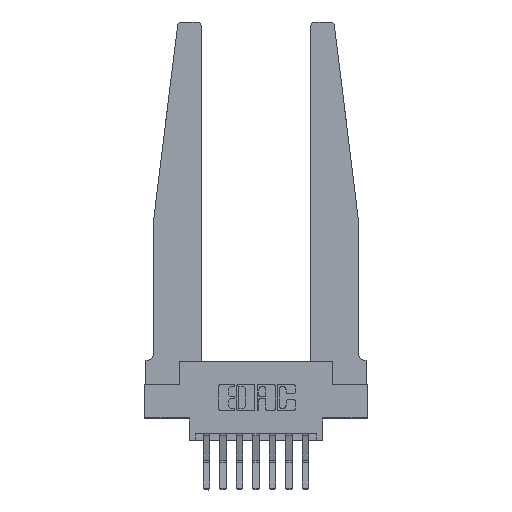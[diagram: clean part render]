
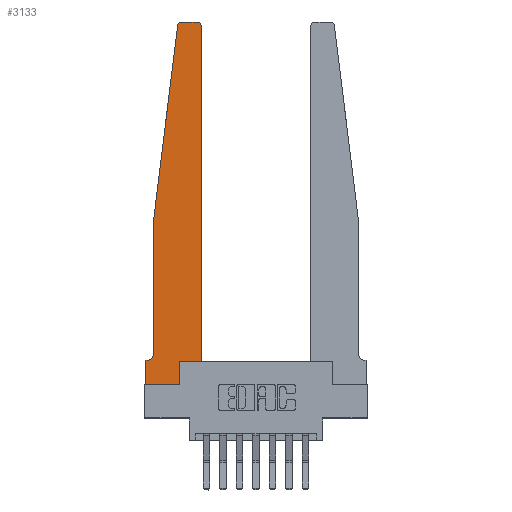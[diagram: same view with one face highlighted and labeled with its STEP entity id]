
A CAD part, top view. The second image highlights one B-rep face of the part: STEP entity #3133.
In plain terms, the highlighted planar face has unit normal (0, 0, 1).
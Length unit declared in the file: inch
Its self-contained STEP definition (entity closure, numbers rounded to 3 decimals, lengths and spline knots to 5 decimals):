
#712 = EDGE_CURVE ( 'NONE', #3959, #6302, #6384, .T. ) ;
#807 = CARTESIAN_POINT ( 'NONE',  ( 0.27653, 2.75, 0.37 ) ) ;
#1016 = CARTESIAN_POINT ( 'NONE',  ( 0.065, 0.2375, 0.37 ) ) ;
#1052 = DIRECTION ( 'NONE',  ( 1., 0., 0. ) ) ;
#1242 = LINE ( 'NONE', #12144, #10127 ) ;
#1416 = VERTEX_POINT ( 'NONE', #8526 ) ;
#1556 = VECTOR ( 'NONE', #14235, 39.37008 ) ;
#1967 = AXIS2_PLACEMENT_3D ( 'NONE', #14248, #7748, #1052 ) ;
#2050 = EDGE_CURVE ( 'NONE', #9724, #7909, #5258, .T. ) ;
#2138 = EDGE_LOOP ( 'NONE', ( #2461, #10904, #9945, #2208, #4222, #2224, #10952, #4134, #10697, #9117, #2568, #9562 ) ) ;
#2208 = ORIENTED_EDGE ( 'NONE', *, *, #712, .T. ) ;
#2224 = ORIENTED_EDGE ( 'NONE', *, *, #2050, .T. ) ;
#2461 = ORIENTED_EDGE ( 'NONE', *, *, #8905, .T. ) ;
#2567 = EDGE_CURVE ( 'NONE', #7302, #8418, #12966, .T. ) ;
#2568 = ORIENTED_EDGE ( 'NONE', *, *, #3024, .T. ) ;
#2835 = CARTESIAN_POINT ( 'NONE',  ( 0.425, 0.18, 0.37 ) ) ;
#2946 = CARTESIAN_POINT ( 'NONE',  ( 0.25, 2.75, 0.37 ) ) ;
#2986 = PLANE ( 'NONE',  #9719 ) ;
#3024 = EDGE_CURVE ( 'NONE', #7614, #8059, #5565, .T. ) ;
#3133 = ADVANCED_FACE ( 'NONE', ( #6787 ), #2986, .T. ) ;
#3278 = EDGE_CURVE ( 'NONE', #8059, #12700, #13773, .T. ) ;
#3384 = VECTOR ( 'NONE', #8274, 39.37008 ) ;
#3524 = AXIS2_PLACEMENT_3D ( 'NONE', #6534, #14160, #7653 ) ;
#3959 = VERTEX_POINT ( 'NONE', #8915 ) ;
#4134 = ORIENTED_EDGE ( 'NONE', *, *, #6622, .T. ) ;
#4147 = DIRECTION ( 'NONE',  ( 0., 0., 1. ) ) ;
#4157 = CARTESIAN_POINT ( 'NONE',  ( 0.015, 0.1875, 0.37 ) ) ;
#4222 = ORIENTED_EDGE ( 'NONE', *, *, #5530, .T. ) ;
#4321 = CARTESIAN_POINT ( 'NONE',  ( 0., 0., 0.37 ) ) ;
#4345 = DIRECTION ( 'NONE',  ( -0.122, -0.992, 0. ) ) ;
#4367 = CARTESIAN_POINT ( 'NONE',  ( 0.065, 0.1875, 0.37 ) ) ;
#4979 = CARTESIAN_POINT ( 'NONE',  ( 0., 0., 0.37 ) ) ;
#5258 = LINE ( 'NONE', #4367, #1556 ) ;
#5395 = CARTESIAN_POINT ( 'NONE',  ( 0.2605, 0.18, 0.37 ) ) ;
#5454 = DIRECTION ( 'NONE',  ( 0., -1., 0. ) ) ;
#5530 = EDGE_CURVE ( 'NONE', #6302, #9724, #9130, .T. ) ;
#5565 = LINE ( 'NONE', #2835, #13611 ) ;
#5891 = CARTESIAN_POINT ( 'NONE',  ( 0.425, 2.72, 0.37 ) ) ;
#6260 = EDGE_CURVE ( 'NONE', #12855, #3959, #11864, .T. ) ;
#6290 = DIRECTION ( 'NONE',  ( 0., 0., -1. ) ) ;
#6302 = VERTEX_POINT ( 'NONE', #1016 ) ;
#6384 = LINE ( 'NONE', #10271, #3384 ) ;
#6534 = CARTESIAN_POINT ( 'NONE',  ( 0.27653, 2.72, 0.37 ) ) ;
#6622 = EDGE_CURVE ( 'NONE', #1416, #7302, #13517, .T. ) ;
#6704 = VECTOR ( 'NONE', #4345, 39.37008 ) ;
#6787 = FACE_OUTER_BOUND ( 'NONE', #2138, .T. ) ;
#6938 = VECTOR ( 'NONE', #5454, 39.37008 ) ;
#7295 = LINE ( 'NONE', #4321, #6938 ) ;
#7302 = VERTEX_POINT ( 'NONE', #12194 ) ;
#7614 = VERTEX_POINT ( 'NONE', #11779 ) ;
#7653 = DIRECTION ( 'NONE',  ( 1., 0., 0. ) ) ;
#7730 = VECTOR ( 'NONE', #11585, 39.37008 ) ;
#7748 = DIRECTION ( 'NONE',  ( 0., 0., 1. ) ) ;
#7772 = EDGE_CURVE ( 'NONE', #8368, #12855, #8424, .T. ) ;
#7803 = DIRECTION ( 'NONE',  ( 1., 0., 0. ) ) ;
#7909 = VERTEX_POINT ( 'NONE', #8936 ) ;
#8059 = VERTEX_POINT ( 'NONE', #5891 ) ;
#8274 = DIRECTION ( 'NONE',  ( 0., -1., 0. ) ) ;
#8368 = VERTEX_POINT ( 'NONE', #807 ) ;
#8418 = VERTEX_POINT ( 'NONE', #10891 ) ;
#8424 = CIRCLE ( 'NONE', #3524, 0.03 ) ;
#8526 = CARTESIAN_POINT ( 'NONE',  ( 0., 0., 0.37 ) ) ;
#8764 = VECTOR ( 'NONE', #10700, 39.37008 ) ;
#8905 = EDGE_CURVE ( 'NONE', #12700, #8368, #11327, .T. ) ;
#8915 = CARTESIAN_POINT ( 'NONE',  ( 0.065, 1.25, 0.37 ) ) ;
#8936 = CARTESIAN_POINT ( 'NONE',  ( 0., 0.1875, 0.37 ) ) ;
#9117 = ORIENTED_EDGE ( 'NONE', *, *, #9867, .T. ) ;
#9130 = CIRCLE ( 'NONE', #9189, 0.05 ) ;
#9189 = AXIS2_PLACEMENT_3D ( 'NONE', #12844, #6290, #13899 ) ;
#9486 = DIRECTION ( 'NONE',  ( 0., 1., 0. ) ) ;
#9562 = ORIENTED_EDGE ( 'NONE', *, *, #3278, .T. ) ;
#9682 = CARTESIAN_POINT ( 'NONE',  ( 0., 0.1875, 0.37 ) ) ;
#9719 = AXIS2_PLACEMENT_3D ( 'NONE', #9682, #4147, #11884 ) ;
#9724 = VERTEX_POINT ( 'NONE', #4157 ) ;
#9829 = CARTESIAN_POINT ( 'NONE',  ( 0.065, 1.25, 0.37 ) ) ;
#9840 = CARTESIAN_POINT ( 'NONE',  ( 0.24675, 2.72367, 0.37 ) ) ;
#9867 = EDGE_CURVE ( 'NONE', #8418, #7614, #1242, .T. ) ;
#9945 = ORIENTED_EDGE ( 'NONE', *, *, #6260, .T. ) ;
#10127 = VECTOR ( 'NONE', #7803, 39.37008 ) ;
#10271 = CARTESIAN_POINT ( 'NONE',  ( 0.065, 1.25, 0.37 ) ) ;
#10421 = VECTOR ( 'NONE', #13054, 39.37008 ) ;
#10697 = ORIENTED_EDGE ( 'NONE', *, *, #2567, .T. ) ;
#10700 = DIRECTION ( 'NONE',  ( -1., 0., 0. ) ) ;
#10755 = CARTESIAN_POINT ( 'NONE',  ( 0.395, 2.75, 0.37 ) ) ;
#10891 = CARTESIAN_POINT ( 'NONE',  ( 0.2605, 0.18, 0.37 ) ) ;
#10904 = ORIENTED_EDGE ( 'NONE', *, *, #7772, .T. ) ;
#10952 = ORIENTED_EDGE ( 'NONE', *, *, #13858, .T. ) ;
#11327 = LINE ( 'NONE', #2946, #8764 ) ;
#11585 = DIRECTION ( 'NONE',  ( 1., 0., 0. ) ) ;
#11779 = CARTESIAN_POINT ( 'NONE',  ( 0.425, 0.18, 0.37 ) ) ;
#11864 = LINE ( 'NONE', #9829, #6704 ) ;
#11884 = DIRECTION ( 'NONE',  ( 1., 0., 0. ) ) ;
#12144 = CARTESIAN_POINT ( 'NONE',  ( 0.425, 0.18, 0.37 ) ) ;
#12194 = CARTESIAN_POINT ( 'NONE',  ( 0.2605, 0., 0.37 ) ) ;
#12700 = VERTEX_POINT ( 'NONE', #10755 ) ;
#12844 = CARTESIAN_POINT ( 'NONE',  ( 0.015, 0.2375, 0.37 ) ) ;
#12855 = VERTEX_POINT ( 'NONE', #9840 ) ;
#12966 = LINE ( 'NONE', #5395, #10421 ) ;
#13054 = DIRECTION ( 'NONE',  ( 0., 1., 0. ) ) ;
#13517 = LINE ( 'NONE', #4979, #7730 ) ;
#13611 = VECTOR ( 'NONE', #9486, 39.37008 ) ;
#13773 = CIRCLE ( 'NONE', #1967, 0.03 ) ;
#13858 = EDGE_CURVE ( 'NONE', #7909, #1416, #7295, .T. ) ;
#13899 = DIRECTION ( 'NONE',  ( -1., 0., 0. ) ) ;
#14160 = DIRECTION ( 'NONE',  ( 0., 0., 1. ) ) ;
#14235 = DIRECTION ( 'NONE',  ( -1., 0., 0. ) ) ;
#14248 = CARTESIAN_POINT ( 'NONE',  ( 0.395, 2.72, 0.37 ) ) ;
